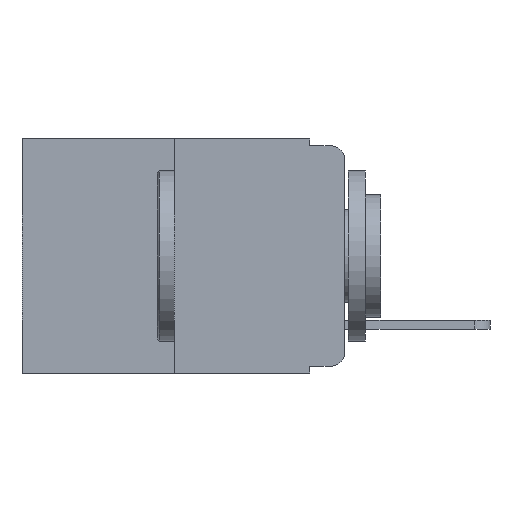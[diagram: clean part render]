
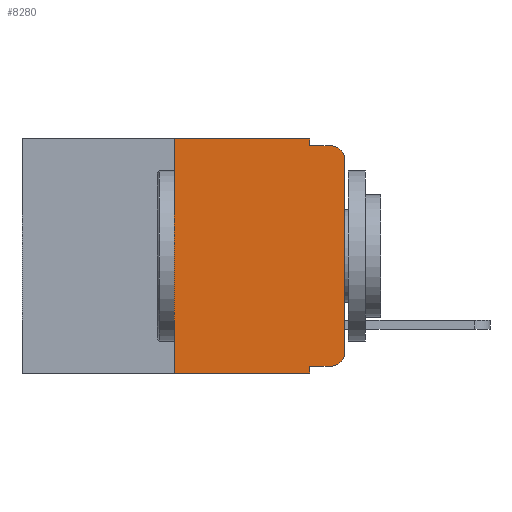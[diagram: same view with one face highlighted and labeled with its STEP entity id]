
A CAD part, left-side view. The second image highlights one B-rep face of the part: STEP entity #8280.
In plain terms, the highlighted planar face has unit normal (-1, 0, 0).
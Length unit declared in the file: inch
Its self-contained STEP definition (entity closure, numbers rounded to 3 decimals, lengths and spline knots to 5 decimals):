
#888 = LINE ( 'NONE', #15816, #17493 ) ;
#1360 = AXIS2_PLACEMENT_3D ( 'NONE', #18769, #14678, #5148 ) ;
#1979 = EDGE_CURVE ( 'NONE', #4538, #12348, #5505, .T. ) ;
#1988 = VERTEX_POINT ( 'NONE', #13283 ) ;
#2023 = LINE ( 'NONE', #19770, #18318 ) ;
#2492 = VERTEX_POINT ( 'NONE', #14593 ) ;
#2606 = FACE_OUTER_BOUND ( 'NONE', #17052, .T. ) ;
#2797 = VERTEX_POINT ( 'NONE', #13046 ) ;
#3336 = PLANE ( 'NONE',  #1360 ) ;
#3636 = CIRCLE ( 'NONE', #18487, 0.02 ) ;
#4046 = DIRECTION ( 'NONE',  ( 0., 0., -1. ) ) ;
#4080 = CARTESIAN_POINT ( 'NONE',  ( 0., 0.051, 0. ) ) ;
#4164 = LINE ( 'NONE', #4187, #16331 ) ;
#4187 = CARTESIAN_POINT ( 'NONE',  ( 0., 0.473, 0. ) ) ;
#4538 = VERTEX_POINT ( 'NONE', #15182 ) ;
#4607 = CARTESIAN_POINT ( 'NONE',  ( 0., 0.25, -0.343 ) ) ;
#4917 = DIRECTION ( 'NONE',  ( 0., -1., 0. ) ) ;
#4948 = EDGE_CURVE ( 'NONE', #8227, #18724, #4164, .T. ) ;
#5148 = DIRECTION ( 'NONE',  ( 0., 0., -1. ) ) ;
#5337 = DIRECTION ( 'NONE',  ( 0., -1., 0. ) ) ;
#5505 = LINE ( 'NONE', #4080, #17367 ) ;
#5616 = CARTESIAN_POINT ( 'NONE',  ( 0., 0.051, -0.333 ) ) ;
#7024 = VERTEX_POINT ( 'NONE', #4607 ) ;
#7389 = EDGE_CURVE ( 'NONE', #2797, #1988, #888, .T. ) ;
#7888 = VECTOR ( 'NONE', #4046, 39.37008 ) ;
#8227 = VERTEX_POINT ( 'NONE', #19843 ) ;
#8280 = ADVANCED_FACE ( 'NONE', ( #2606 ), #3336, .F. ) ;
#8644 = EDGE_CURVE ( 'NONE', #10869, #17465, #2023, .T. ) ;
#8848 = CARTESIAN_POINT ( 'NONE',  ( 0., 0.02, -0.03 ) ) ;
#9689 = ORIENTED_EDGE ( 'NONE', *, *, #8644, .T. ) ;
#9715 = VECTOR ( 'NONE', #17544, 39.37008 ) ;
#9833 = ORIENTED_EDGE ( 'NONE', *, *, #10372, .T. ) ;
#9903 = CARTESIAN_POINT ( 'NONE',  ( 0., 0.02, -0.313 ) ) ;
#9960 = LINE ( 'NONE', #5616, #13513 ) ;
#10114 = CARTESIAN_POINT ( 'NONE',  ( 0., 0.051, 0. ) ) ;
#10118 = ORIENTED_EDGE ( 'NONE', *, *, #7389, .F. ) ;
#10203 = ORIENTED_EDGE ( 'NONE', *, *, #11830, .F. ) ;
#10372 = EDGE_CURVE ( 'NONE', #17465, #1988, #3636, .T. ) ;
#10483 = DIRECTION ( 'NONE',  ( 0., 0., -1. ) ) ;
#10616 = ORIENTED_EDGE ( 'NONE', *, *, #4948, .F. ) ;
#10869 = VERTEX_POINT ( 'NONE', #16911 ) ;
#10996 = EDGE_CURVE ( 'NONE', #7024, #12348, #17800, .T. ) ;
#11010 = ORIENTED_EDGE ( 'NONE', *, *, #11570, .F. ) ;
#11095 = CARTESIAN_POINT ( 'NONE',  ( 0., 0., -0.03 ) ) ;
#11436 = DIRECTION ( 'NONE',  ( 0., 0., 1. ) ) ;
#11493 = DIRECTION ( 'NONE',  ( 0., 0., -1. ) ) ;
#11570 = EDGE_CURVE ( 'NONE', #7024, #8227, #13300, .T. ) ;
#11745 = EDGE_CURVE ( 'NONE', #4538, #2492, #9960, .T. ) ;
#11753 = ORIENTED_EDGE ( 'NONE', *, *, #10996, .T. ) ;
#11830 = EDGE_CURVE ( 'NONE', #18724, #2797, #19520, .T. ) ;
#11848 = ORIENTED_EDGE ( 'NONE', *, *, #1979, .F. ) ;
#12253 = ORIENTED_EDGE ( 'NONE', *, *, #11745, .T. ) ;
#12348 = VERTEX_POINT ( 'NONE', #16265 ) ;
#12828 = ORIENTED_EDGE ( 'NONE', *, *, #18188, .T. ) ;
#13046 = CARTESIAN_POINT ( 'NONE',  ( 0., 0.051, -0.01 ) ) ;
#13055 = DIRECTION ( 'NONE',  ( 0., 0., -1. ) ) ;
#13283 = CARTESIAN_POINT ( 'NONE',  ( 0., 0.02, -0.01 ) ) ;
#13300 = LINE ( 'NONE', #14632, #9715 ) ;
#13513 = VECTOR ( 'NONE', #19140, 39.37008 ) ;
#13779 = CARTESIAN_POINT ( 'NONE',  ( 0., 0.051, 0. ) ) ;
#14493 = CARTESIAN_POINT ( 'NONE',  ( 0., 0.473, -0.343 ) ) ;
#14593 = CARTESIAN_POINT ( 'NONE',  ( 0., 0.02, -0.333 ) ) ;
#14632 = CARTESIAN_POINT ( 'NONE',  ( 0., 0.25, 0. ) ) ;
#14678 = DIRECTION ( 'NONE',  ( 1., 0., 0. ) ) ;
#15182 = CARTESIAN_POINT ( 'NONE',  ( 0., 0.051, -0.333 ) ) ;
#15315 = AXIS2_PLACEMENT_3D ( 'NONE', #9903, #19819, #11493 ) ;
#15816 = CARTESIAN_POINT ( 'NONE',  ( 0., 0.051, -0.01 ) ) ;
#16265 = CARTESIAN_POINT ( 'NONE',  ( 0., 0.051, -0.343 ) ) ;
#16331 = VECTOR ( 'NONE', #5337, 39.37008 ) ;
#16911 = CARTESIAN_POINT ( 'NONE',  ( 0., 0., -0.313 ) ) ;
#17052 = EDGE_LOOP ( 'NONE', ( #9689, #9833, #10118, #10203, #10616, #11010, #11753, #11848, #12253, #12828 ) ) ;
#17247 = DIRECTION ( 'NONE',  ( 0., -1., 0. ) ) ;
#17367 = VECTOR ( 'NONE', #13055, 39.37008 ) ;
#17390 = VECTOR ( 'NONE', #4917, 39.37008 ) ;
#17465 = VERTEX_POINT ( 'NONE', #11095 ) ;
#17493 = VECTOR ( 'NONE', #17247, 39.37008 ) ;
#17544 = DIRECTION ( 'NONE',  ( 0., 0., 1. ) ) ;
#17800 = LINE ( 'NONE', #14493, #17390 ) ;
#18188 = EDGE_CURVE ( 'NONE', #2492, #10869, #18458, .T. ) ;
#18318 = VECTOR ( 'NONE', #11436, 39.37008 ) ;
#18458 = CIRCLE ( 'NONE', #15315, 0.02 ) ;
#18487 = AXIS2_PLACEMENT_3D ( 'NONE', #8848, #19021, #10483 ) ;
#18724 = VERTEX_POINT ( 'NONE', #10114 ) ;
#18769 = CARTESIAN_POINT ( 'NONE',  ( 0., 0.473, 0. ) ) ;
#19021 = DIRECTION ( 'NONE',  ( -1., 0., 0. ) ) ;
#19140 = DIRECTION ( 'NONE',  ( 0., -1., 0. ) ) ;
#19520 = LINE ( 'NONE', #13779, #7888 ) ;
#19770 = CARTESIAN_POINT ( 'NONE',  ( 0., 0., 0. ) ) ;
#19819 = DIRECTION ( 'NONE',  ( -1., 0., 0. ) ) ;
#19843 = CARTESIAN_POINT ( 'NONE',  ( 0., 0.25, 0. ) ) ;
